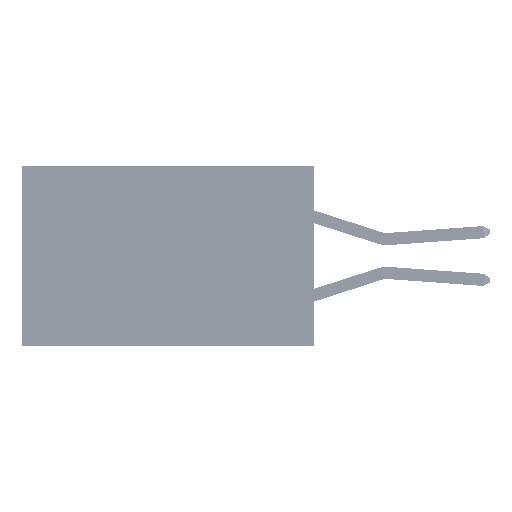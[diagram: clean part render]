
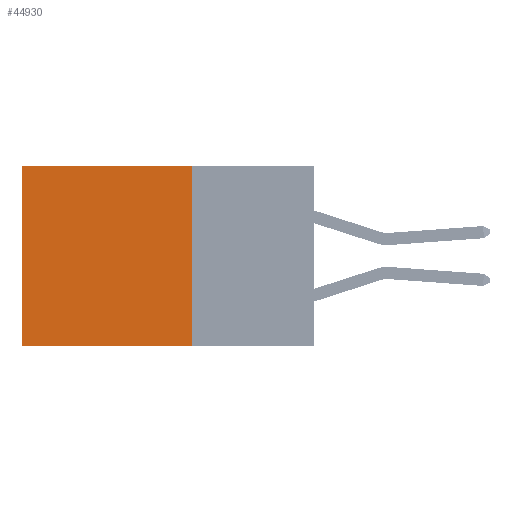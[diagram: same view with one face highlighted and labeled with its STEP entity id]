
A CAD part, left-side view. The second image highlights one B-rep face of the part: STEP entity #44930.
In plain terms, the highlighted planar face has unit normal (-1, 0, 0).
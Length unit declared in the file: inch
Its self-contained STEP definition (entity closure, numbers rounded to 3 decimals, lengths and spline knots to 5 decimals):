
#250 = LINE ( 'NONE', #19137, #1224 ) ;
#340 = CARTESIAN_POINT ( 'NONE',  ( 0.2875, 0.25, 0. ) ) ;
#1224 = VECTOR ( 'NONE', #22598, 39.37008 ) ;
#1934 = CARTESIAN_POINT ( 'NONE',  ( 0.2875, 0.25, 0. ) ) ;
#2196 = EDGE_LOOP ( 'NONE', ( #42174, #35703, #22310, #39088 ) ) ;
#5395 = DIRECTION ( 'NONE',  ( 0., 1., 0. ) ) ;
#7480 = EDGE_CURVE ( 'NONE', #42681, #27344, #38271, .T. ) ;
#8153 = VECTOR ( 'NONE', #5395, 39.37008 ) ;
#8906 = CARTESIAN_POINT ( 'NONE',  ( 0.2875, 0.25, -0.37 ) ) ;
#9391 = FACE_OUTER_BOUND ( 'NONE', #2196, .T. ) ;
#9906 = VECTOR ( 'NONE', #20225, 39.37008 ) ;
#10107 = PLANE ( 'NONE',  #35206 ) ;
#13294 = VERTEX_POINT ( 'NONE', #19824 ) ;
#13538 = CARTESIAN_POINT ( 'NONE',  ( 0.2875, 0.25, 0. ) ) ;
#14717 = CARTESIAN_POINT ( 'NONE',  ( 0.2875, 0.6, 0. ) ) ;
#16640 = EDGE_CURVE ( 'NONE', #27344, #28451, #37537, .T. ) ;
#17005 = LINE ( 'NONE', #8906, #9906 ) ;
#18019 = EDGE_CURVE ( 'NONE', #42681, #13294, #250, .T. ) ;
#19128 = DIRECTION ( 'NONE',  ( 0., 0., -1. ) ) ;
#19137 = CARTESIAN_POINT ( 'NONE',  ( 0.2875, 0.25, 0. ) ) ;
#19824 = CARTESIAN_POINT ( 'NONE',  ( 0.2875, 0.25, -0.37 ) ) ;
#20225 = DIRECTION ( 'NONE',  ( 0., 1., 0. ) ) ;
#20443 = DIRECTION ( 'NONE',  ( 1., 0., 0. ) ) ;
#22310 = ORIENTED_EDGE ( 'NONE', *, *, #18019, .F. ) ;
#22598 = DIRECTION ( 'NONE',  ( 0., 0., -1. ) ) ;
#24124 = DIRECTION ( 'NONE',  ( 0., 0., -1. ) ) ;
#27344 = VERTEX_POINT ( 'NONE', #14717 ) ;
#28451 = VERTEX_POINT ( 'NONE', #35327 ) ;
#29460 = CARTESIAN_POINT ( 'NONE',  ( 0.2875, 0.6, 0. ) ) ;
#29465 = EDGE_CURVE ( 'NONE', #13294, #28451, #17005, .T. ) ;
#35206 = AXIS2_PLACEMENT_3D ( 'NONE', #13538, #20443, #24124 ) ;
#35327 = CARTESIAN_POINT ( 'NONE',  ( 0.2875, 0.6, -0.37 ) ) ;
#35703 = ORIENTED_EDGE ( 'NONE', *, *, #29465, .F. ) ;
#37537 = LINE ( 'NONE', #29460, #40277 ) ;
#38271 = LINE ( 'NONE', #1934, #8153 ) ;
#39088 = ORIENTED_EDGE ( 'NONE', *, *, #7480, .T. ) ;
#40277 = VECTOR ( 'NONE', #19128, 39.37008 ) ;
#42174 = ORIENTED_EDGE ( 'NONE', *, *, #16640, .T. ) ;
#42681 = VERTEX_POINT ( 'NONE', #340 ) ;
#44930 = ADVANCED_FACE ( 'NONE', ( #9391 ), #10107, .F. ) ;
